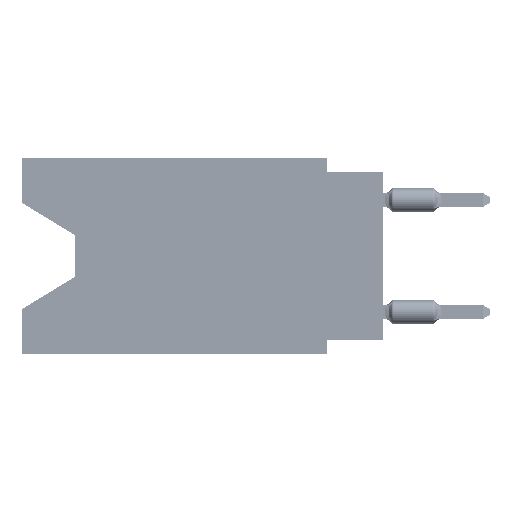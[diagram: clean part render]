
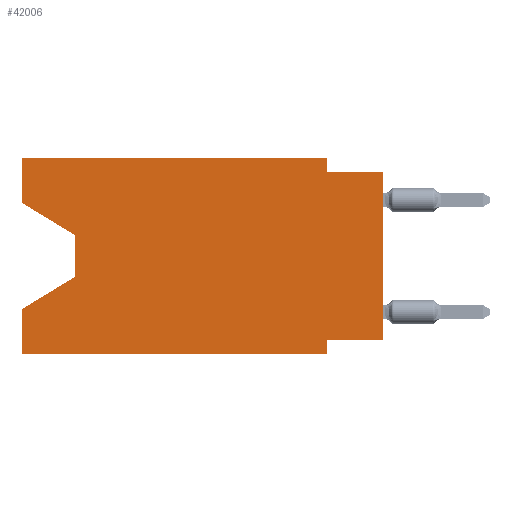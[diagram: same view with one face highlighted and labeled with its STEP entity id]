
A CAD part, left-side view. The second image highlights one B-rep face of the part: STEP entity #42006.
In plain terms, the highlighted planar face has unit normal (-1, 0, 0).
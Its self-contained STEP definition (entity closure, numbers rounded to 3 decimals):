
#268 = CARTESIAN_POINT ( 'NONE',  ( 0., 13.97, -3.505 ) ) ;
#510 = VECTOR ( 'NONE', #34953, 1000. ) ;
#572 = EDGE_CURVE ( 'NONE', #19238, #6424, #40699, .T. ) ;
#2612 = VECTOR ( 'NONE', #7338, 1000. ) ;
#3398 = CARTESIAN_POINT ( 'NONE',  ( 0., 0., -0.635 ) ) ;
#4535 = VERTEX_POINT ( 'NONE', #28072 ) ;
#5222 = DIRECTION ( 'NONE',  ( 1., 0., 0. ) ) ;
#6269 = ORIENTED_EDGE ( 'NONE', *, *, #28296, .F. ) ;
#6424 = VERTEX_POINT ( 'NONE', #72040 ) ;
#7338 = DIRECTION ( 'NONE',  ( 0., 0., 1. ) ) ;
#7784 = EDGE_CURVE ( 'NONE', #29259, #15127, #25944, .T. ) ;
#9220 = LINE ( 'NONE', #66634, #47595 ) ;
#10848 = LINE ( 'NONE', #29267, #44293 ) ;
#12055 = FACE_OUTER_BOUND ( 'NONE', #29135, .T. ) ;
#15127 = VERTEX_POINT ( 'NONE', #79492 ) ;
#15283 = LINE ( 'NONE', #41406, #16386 ) ;
#16386 = VECTOR ( 'NONE', #24977, 1000. ) ;
#16700 = CARTESIAN_POINT ( 'NONE',  ( 0., 2.54, -8.255 ) ) ;
#18609 = CARTESIAN_POINT ( 'NONE',  ( 0., 0., -8.255 ) ) ;
#19238 = VERTEX_POINT ( 'NONE', #66407 ) ;
#19512 = CARTESIAN_POINT ( 'NONE',  ( 0., 13.97, -3.505 ) ) ;
#21190 = VERTEX_POINT ( 'NONE', #59785 ) ;
#21792 = VERTEX_POINT ( 'NONE', #16700 ) ;
#23149 = ORIENTED_EDGE ( 'NONE', *, *, #60565, .F. ) ;
#24977 = DIRECTION ( 'NONE',  ( 0., -0.855, -0.519 ) ) ;
#25005 = VECTOR ( 'NONE', #32308, 1000. ) ;
#25944 = LINE ( 'NONE', #268, #67487 ) ;
#27724 = EDGE_CURVE ( 'NONE', #69754, #29259, #15283, .T. ) ;
#28072 = CARTESIAN_POINT ( 'NONE',  ( 0., 2.54, -8.89 ) ) ;
#28296 = EDGE_CURVE ( 'NONE', #69754, #33045, #32562, .T. ) ;
#29135 = EDGE_LOOP ( 'NONE', ( #37372, #49455, #39261, #48295, #33677, #23149, #68133, #33555, #33306, #46522, #64427, #6269 ) ) ;
#29259 = VERTEX_POINT ( 'NONE', #19512 ) ;
#29267 = CARTESIAN_POINT ( 'NONE',  ( 0., 0., 0. ) ) ;
#30097 = VECTOR ( 'NONE', #39722, 1000. ) ;
#30137 = VECTOR ( 'NONE', #71565, 1000. ) ;
#31348 = VERTEX_POINT ( 'NONE', #68064 ) ;
#32308 = DIRECTION ( 'NONE',  ( 0., 1., 0. ) ) ;
#32443 = CARTESIAN_POINT ( 'NONE',  ( 0., 2.54, 0. ) ) ;
#32562 = LINE ( 'NONE', #59968, #30137 ) ;
#33045 = VERTEX_POINT ( 'NONE', #74084 ) ;
#33306 = ORIENTED_EDGE ( 'NONE', *, *, #50113, .F. ) ;
#33513 = VECTOR ( 'NONE', #61638, 1000. ) ;
#33555 = ORIENTED_EDGE ( 'NONE', *, *, #71893, .T. ) ;
#33677 = ORIENTED_EDGE ( 'NONE', *, *, #71328, .T. ) ;
#34953 = DIRECTION ( 'NONE',  ( 0., -1., 0. ) ) ;
#35241 = EDGE_CURVE ( 'NONE', #15127, #6424, #48776, .T. ) ;
#36927 = CARTESIAN_POINT ( 'NONE',  ( 0., 16.383, 0. ) ) ;
#37372 = ORIENTED_EDGE ( 'NONE', *, *, #27724, .T. ) ;
#38216 = AXIS2_PLACEMENT_3D ( 'NONE', #36927, #5222, #76754 ) ;
#39083 = VECTOR ( 'NONE', #60790, 1000. ) ;
#39261 = ORIENTED_EDGE ( 'NONE', *, *, #35241, .T. ) ;
#39641 = LINE ( 'NONE', #66203, #54152 ) ;
#39722 = DIRECTION ( 'NONE',  ( 0., 0., -1. ) ) ;
#40699 = LINE ( 'NONE', #66009, #2612 ) ;
#41406 = CARTESIAN_POINT ( 'NONE',  ( 0., 16.383, -2.038 ) ) ;
#41758 = DIRECTION ( 'NONE',  ( 0., -1., 0. ) ) ;
#42006 = ADVANCED_FACE ( 'NONE', ( #12055 ), #56632, .F. ) ;
#43882 = LINE ( 'NONE', #18609, #25005 ) ;
#44293 = VECTOR ( 'NONE', #75115, 1000. ) ;
#46522 = ORIENTED_EDGE ( 'NONE', *, *, #53632, .F. ) ;
#47595 = VECTOR ( 'NONE', #41758, 1000. ) ;
#47799 = EDGE_CURVE ( 'NONE', #31348, #21792, #43882, .T. ) ;
#48295 = ORIENTED_EDGE ( 'NONE', *, *, #572, .F. ) ;
#48776 = LINE ( 'NONE', #67643, #39083 ) ;
#49455 = ORIENTED_EDGE ( 'NONE', *, *, #7784, .T. ) ;
#50113 = EDGE_CURVE ( 'NONE', #84137, #21190, #80913, .T. ) ;
#53632 = EDGE_CURVE ( 'NONE', #60664, #84137, #66285, .T. ) ;
#54152 = VECTOR ( 'NONE', #58932, 1000. ) ;
#55084 = CARTESIAN_POINT ( 'NONE',  ( 0., 16.383, -8.89 ) ) ;
#56632 = PLANE ( 'NONE',  #38216 ) ;
#58932 = DIRECTION ( 'NONE',  ( 0., 0., -1. ) ) ;
#59785 = CARTESIAN_POINT ( 'NONE',  ( 0., 0., -0.635 ) ) ;
#59968 = CARTESIAN_POINT ( 'NONE',  ( 0., 16.383, 0. ) ) ;
#60565 = EDGE_CURVE ( 'NONE', #21792, #4535, #39641, .T. ) ;
#60664 = VERTEX_POINT ( 'NONE', #81160 ) ;
#60790 = DIRECTION ( 'NONE',  ( 0., 0.855, -0.519 ) ) ;
#61638 = DIRECTION ( 'NONE',  ( 0., -1., 0. ) ) ;
#64427 = ORIENTED_EDGE ( 'NONE', *, *, #83981, .F. ) ;
#65742 = CARTESIAN_POINT ( 'NONE',  ( 0., 16.383, -2.038 ) ) ;
#65927 = LINE ( 'NONE', #55084, #510 ) ;
#66009 = CARTESIAN_POINT ( 'NONE',  ( 0., 16.383, 0. ) ) ;
#66203 = CARTESIAN_POINT ( 'NONE',  ( 0., 2.54, -8.89 ) ) ;
#66285 = LINE ( 'NONE', #32443, #30097 ) ;
#66407 = CARTESIAN_POINT ( 'NONE',  ( 0., 16.383, -8.89 ) ) ;
#66634 = CARTESIAN_POINT ( 'NONE',  ( 0., 16.383, 0. ) ) ;
#67487 = VECTOR ( 'NONE', #73055, 1000. ) ;
#67643 = CARTESIAN_POINT ( 'NONE',  ( 0., 13.97, -5.385 ) ) ;
#68064 = CARTESIAN_POINT ( 'NONE',  ( 0., 0., -8.255 ) ) ;
#68133 = ORIENTED_EDGE ( 'NONE', *, *, #47799, .F. ) ;
#69585 = CARTESIAN_POINT ( 'NONE',  ( 0., 2.54, -0.635 ) ) ;
#69754 = VERTEX_POINT ( 'NONE', #65742 ) ;
#71328 = EDGE_CURVE ( 'NONE', #19238, #4535, #65927, .T. ) ;
#71565 = DIRECTION ( 'NONE',  ( 0., 0., 1. ) ) ;
#71893 = EDGE_CURVE ( 'NONE', #31348, #21190, #10848, .T. ) ;
#72040 = CARTESIAN_POINT ( 'NONE',  ( 0., 16.383, -6.852 ) ) ;
#73055 = DIRECTION ( 'NONE',  ( 0., 0., -1. ) ) ;
#74084 = CARTESIAN_POINT ( 'NONE',  ( 0., 16.383, 0. ) ) ;
#75115 = DIRECTION ( 'NONE',  ( 0., 0., 1. ) ) ;
#76754 = DIRECTION ( 'NONE',  ( 0., 0., -1. ) ) ;
#79492 = CARTESIAN_POINT ( 'NONE',  ( 0., 13.97, -5.385 ) ) ;
#80913 = LINE ( 'NONE', #3398, #33513 ) ;
#81160 = CARTESIAN_POINT ( 'NONE',  ( 0., 2.54, 0. ) ) ;
#83981 = EDGE_CURVE ( 'NONE', #33045, #60664, #9220, .T. ) ;
#84137 = VERTEX_POINT ( 'NONE', #69585 ) ;
